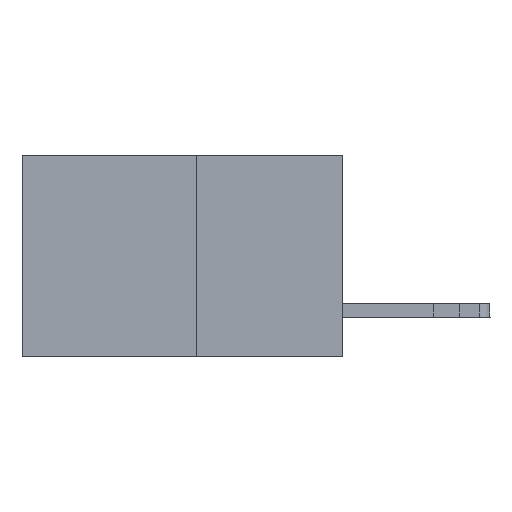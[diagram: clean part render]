
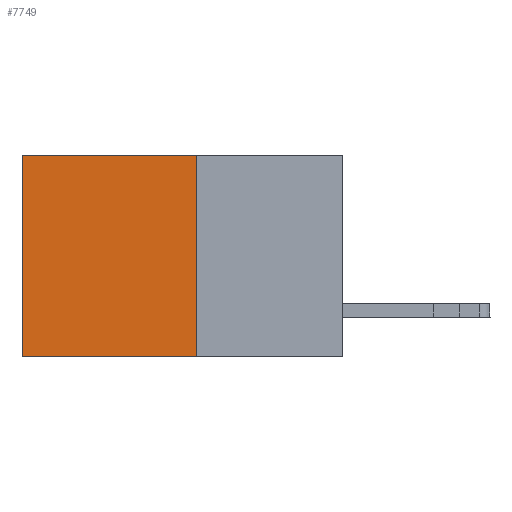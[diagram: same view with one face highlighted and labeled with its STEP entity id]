
A CAD part, left-side view. The second image highlights one B-rep face of the part: STEP entity #7749.
In plain terms, the highlighted planar face has unit normal (-1, 0, 0).
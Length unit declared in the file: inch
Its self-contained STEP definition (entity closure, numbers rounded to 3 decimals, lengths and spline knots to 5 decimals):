
#137 = LINE ( 'NONE', #16966, #9777 ) ;
#1720 = CARTESIAN_POINT ( 'NONE',  ( 0.277, 0.27, -0.37 ) ) ;
#2304 = EDGE_CURVE ( 'NONE', #19794, #4921, #8830, .T. ) ;
#2980 = DIRECTION ( 'NONE',  ( 0., 1., 0. ) ) ;
#3019 = DIRECTION ( 'NONE',  ( 0., 0., -1. ) ) ;
#3422 = PLANE ( 'NONE',  #18231 ) ;
#4921 = VERTEX_POINT ( 'NONE', #10666 ) ;
#5225 = FACE_OUTER_BOUND ( 'NONE', #5447, .T. ) ;
#5447 = EDGE_LOOP ( 'NONE', ( #14577, #20081, #6040, #11673 ) ) ;
#6040 = ORIENTED_EDGE ( 'NONE', *, *, #8741, .F. ) ;
#6391 = CARTESIAN_POINT ( 'NONE',  ( 0.277, 0.59, -0.37 ) ) ;
#7749 = ADVANCED_FACE ( 'NONE', ( #5225 ), #3422, .F. ) ;
#8741 = EDGE_CURVE ( 'NONE', #21529, #19794, #137, .T. ) ;
#8830 = LINE ( 'NONE', #16189, #23541 ) ;
#9777 = VECTOR ( 'NONE', #22177, 39.37008 ) ;
#10666 = CARTESIAN_POINT ( 'NONE',  ( 0.277, 0.59, -0.37 ) ) ;
#11673 = ORIENTED_EDGE ( 'NONE', *, *, #22738, .T. ) ;
#11915 = CARTESIAN_POINT ( 'NONE',  ( 0.277, 0.59, 0. ) ) ;
#11928 = LINE ( 'NONE', #6391, #13852 ) ;
#12120 = CARTESIAN_POINT ( 'NONE',  ( 0.277, 0.27, 0. ) ) ;
#12155 = EDGE_CURVE ( 'NONE', #13308, #4921, #11928, .T. ) ;
#13308 = VERTEX_POINT ( 'NONE', #11915 ) ;
#13570 = CARTESIAN_POINT ( 'NONE',  ( 0.277, 0.27, 0. ) ) ;
#13852 = VECTOR ( 'NONE', #3019, 39.37008 ) ;
#14050 = LINE ( 'NONE', #12120, #14827 ) ;
#14577 = ORIENTED_EDGE ( 'NONE', *, *, #12155, .T. ) ;
#14827 = VECTOR ( 'NONE', #2980, 39.37008 ) ;
#16189 = CARTESIAN_POINT ( 'NONE',  ( 0.277, 0.27, -0.37 ) ) ;
#16296 = DIRECTION ( 'NONE',  ( 0., 0., -1. ) ) ;
#16966 = CARTESIAN_POINT ( 'NONE',  ( 0.277, 0.27, -0.37 ) ) ;
#18231 = AXIS2_PLACEMENT_3D ( 'NONE', #23539, #22102, #16296 ) ;
#19794 = VERTEX_POINT ( 'NONE', #1720 ) ;
#20081 = ORIENTED_EDGE ( 'NONE', *, *, #2304, .F. ) ;
#21529 = VERTEX_POINT ( 'NONE', #13570 ) ;
#22102 = DIRECTION ( 'NONE',  ( 1., 0., 0. ) ) ;
#22177 = DIRECTION ( 'NONE',  ( 0., 0., -1. ) ) ;
#22738 = EDGE_CURVE ( 'NONE', #21529, #13308, #14050, .T. ) ;
#23539 = CARTESIAN_POINT ( 'NONE',  ( 0.277, 0.27, -0.37 ) ) ;
#23541 = VECTOR ( 'NONE', #23761, 39.37008 ) ;
#23761 = DIRECTION ( 'NONE',  ( 0., 1., 0. ) ) ;
